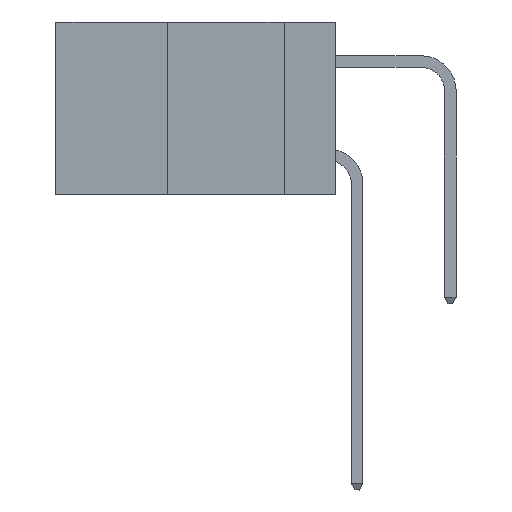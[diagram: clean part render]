
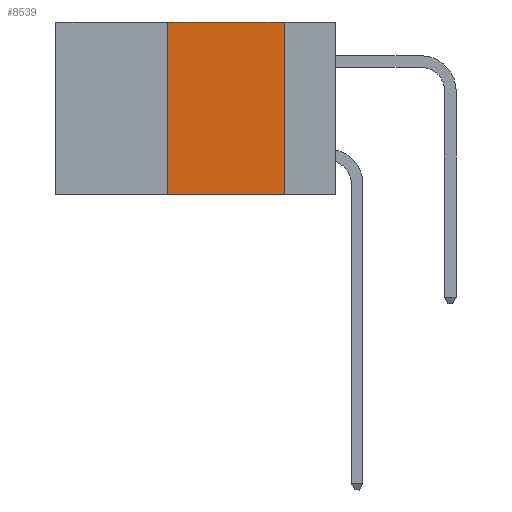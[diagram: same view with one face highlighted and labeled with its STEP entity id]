
A CAD part, left-side view. The second image highlights one B-rep face of the part: STEP entity #8539.
In plain terms, the highlighted planar face has unit normal (-1, 0, 0).
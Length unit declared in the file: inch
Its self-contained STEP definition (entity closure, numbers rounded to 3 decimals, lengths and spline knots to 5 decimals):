
#808 = FACE_OUTER_BOUND ( 'NONE', #7539, .T. ) ;
#1485 = LINE ( 'NONE', #25198, #22094 ) ;
#1857 = DIRECTION ( 'NONE',  ( 0., 0., 1. ) ) ;
#2529 = VECTOR ( 'NONE', #22431, 39.37008 ) ;
#4758 = DIRECTION ( 'NONE',  ( 1., 0., 0. ) ) ;
#5209 = VECTOR ( 'NONE', #10123, 39.37008 ) ;
#6010 = CARTESIAN_POINT ( 'NONE',  ( 0., 0.6, 0. ) ) ;
#6105 = VECTOR ( 'NONE', #23459, 39.37008 ) ;
#6690 = LINE ( 'NONE', #14553, #2529 ) ;
#7539 = EDGE_LOOP ( 'NONE', ( #9965, #9151, #18263, #23209 ) ) ;
#8514 = PLANE ( 'NONE',  #14723 ) ;
#8539 = ADVANCED_FACE ( 'NONE', ( #808 ), #8514, .F. ) ;
#9151 = ORIENTED_EDGE ( 'NONE', *, *, #23814, .F. ) ;
#9872 = LINE ( 'NONE', #6010, #5209 ) ;
#9965 = ORIENTED_EDGE ( 'NONE', *, *, #25021, .F. ) ;
#10123 = DIRECTION ( 'NONE',  ( 0., -1., 0. ) ) ;
#10469 = VERTEX_POINT ( 'NONE', #25414 ) ;
#10722 = EDGE_CURVE ( 'NONE', #21219, #13686, #6690, .T. ) ;
#11052 = LINE ( 'NONE', #15060, #6105 ) ;
#11827 = EDGE_CURVE ( 'NONE', #21219, #16424, #1485, .T. ) ;
#13686 = VERTEX_POINT ( 'NONE', #13808 ) ;
#13808 = CARTESIAN_POINT ( 'NONE',  ( 0., 0.11, -0.37 ) ) ;
#14553 = CARTESIAN_POINT ( 'NONE',  ( 0., 0.6, -0.37 ) ) ;
#14723 = AXIS2_PLACEMENT_3D ( 'NONE', #22331, #4758, #20395 ) ;
#15060 = CARTESIAN_POINT ( 'NONE',  ( 0., 0.11, 0. ) ) ;
#16424 = VERTEX_POINT ( 'NONE', #23739 ) ;
#18263 = ORIENTED_EDGE ( 'NONE', *, *, #11827, .F. ) ;
#20395 = DIRECTION ( 'NONE',  ( 0., 0., -1. ) ) ;
#21219 = VERTEX_POINT ( 'NONE', #23544 ) ;
#22094 = VECTOR ( 'NONE', #1857, 39.37008 ) ;
#22331 = CARTESIAN_POINT ( 'NONE',  ( 0., 0.6, 0. ) ) ;
#22431 = DIRECTION ( 'NONE',  ( 0., -1., 0. ) ) ;
#23209 = ORIENTED_EDGE ( 'NONE', *, *, #10722, .T. ) ;
#23459 = DIRECTION ( 'NONE',  ( 0., 0., -1. ) ) ;
#23544 = CARTESIAN_POINT ( 'NONE',  ( 0., 0.36, -0.37 ) ) ;
#23739 = CARTESIAN_POINT ( 'NONE',  ( 0., 0.36, 0. ) ) ;
#23814 = EDGE_CURVE ( 'NONE', #16424, #10469, #9872, .T. ) ;
#25021 = EDGE_CURVE ( 'NONE', #10469, #13686, #11052, .T. ) ;
#25198 = CARTESIAN_POINT ( 'NONE',  ( 0., 0.36, 0. ) ) ;
#25414 = CARTESIAN_POINT ( 'NONE',  ( 0., 0.11, 0. ) ) ;
